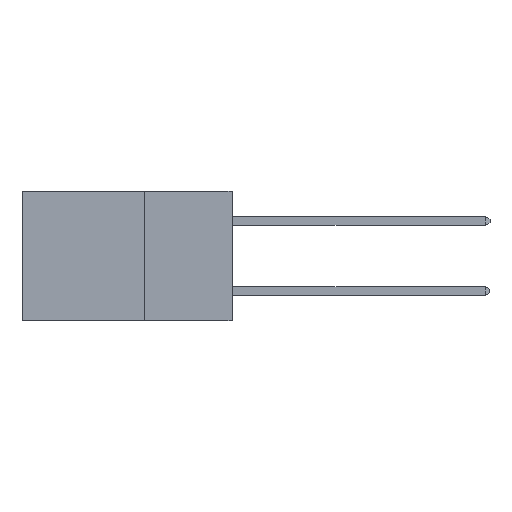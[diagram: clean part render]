
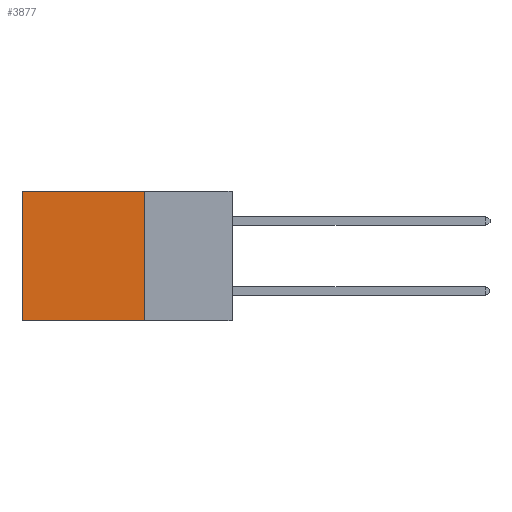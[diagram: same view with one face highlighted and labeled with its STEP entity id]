
A CAD part, left-side view. The second image highlights one B-rep face of the part: STEP entity #3877.
In plain terms, the highlighted planar face has unit normal (-1, 0, 0).
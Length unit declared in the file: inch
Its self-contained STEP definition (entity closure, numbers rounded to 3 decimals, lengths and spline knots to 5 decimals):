
#20 = VECTOR ( 'NONE', #9128, 39.37008 ) ;
#154 = VECTOR ( 'NONE', #14151, 39.37008 ) ;
#423 = LINE ( 'NONE', #7875, #20 ) ;
#1464 = ORIENTED_EDGE ( 'NONE', *, *, #12801, .F. ) ;
#1496 = EDGE_CURVE ( 'NONE', #2145, #12539, #3213, .T. ) ;
#2145 = VERTEX_POINT ( 'NONE', #14210 ) ;
#2491 = VECTOR ( 'NONE', #6498, 39.37008 ) ;
#3213 = LINE ( 'NONE', #7158, #15294 ) ;
#3415 = VERTEX_POINT ( 'NONE', #4336 ) ;
#3877 = ADVANCED_FACE ( 'NONE', ( #12768 ), #14203, .F. ) ;
#4336 = CARTESIAN_POINT ( 'NONE',  ( 0.2875, 0.25, 0. ) ) ;
#5233 = AXIS2_PLACEMENT_3D ( 'NONE', #11856, #15379, #8330 ) ;
#5775 = CARTESIAN_POINT ( 'NONE',  ( 0.2875, 0.6, 0. ) ) ;
#6446 = EDGE_CURVE ( 'NONE', #3415, #8809, #423, .T. ) ;
#6498 = DIRECTION ( 'NONE',  ( 0., 0., -1. ) ) ;
#7106 = DIRECTION ( 'NONE',  ( 0., 1., 0. ) ) ;
#7158 = CARTESIAN_POINT ( 'NONE',  ( 0.2875, 0.25, -0.37 ) ) ;
#7875 = CARTESIAN_POINT ( 'NONE',  ( 0.2875, 0.25, 0. ) ) ;
#8330 = DIRECTION ( 'NONE',  ( 0., 0., -1. ) ) ;
#8809 = VERTEX_POINT ( 'NONE', #14039 ) ;
#8878 = EDGE_CURVE ( 'NONE', #8809, #12539, #13314, .T. ) ;
#9128 = DIRECTION ( 'NONE',  ( 0., 1., 0. ) ) ;
#11319 = CARTESIAN_POINT ( 'NONE',  ( 0.2875, 0.25, 0. ) ) ;
#11384 = ORIENTED_EDGE ( 'NONE', *, *, #1496, .F. ) ;
#11856 = CARTESIAN_POINT ( 'NONE',  ( 0.2875, 0.25, 0. ) ) ;
#12539 = VERTEX_POINT ( 'NONE', #13288 ) ;
#12768 = FACE_OUTER_BOUND ( 'NONE', #15483, .T. ) ;
#12801 = EDGE_CURVE ( 'NONE', #3415, #2145, #15418, .T. ) ;
#13288 = CARTESIAN_POINT ( 'NONE',  ( 0.2875, 0.6, -0.37 ) ) ;
#13314 = LINE ( 'NONE', #5775, #154 ) ;
#14039 = CARTESIAN_POINT ( 'NONE',  ( 0.2875, 0.6, 0. ) ) ;
#14120 = ORIENTED_EDGE ( 'NONE', *, *, #6446, .T. ) ;
#14151 = DIRECTION ( 'NONE',  ( 0., 0., -1. ) ) ;
#14203 = PLANE ( 'NONE',  #5233 ) ;
#14210 = CARTESIAN_POINT ( 'NONE',  ( 0.2875, 0.25, -0.37 ) ) ;
#14860 = ORIENTED_EDGE ( 'NONE', *, *, #8878, .T. ) ;
#15294 = VECTOR ( 'NONE', #7106, 39.37008 ) ;
#15379 = DIRECTION ( 'NONE',  ( 1., 0., 0. ) ) ;
#15418 = LINE ( 'NONE', #11319, #2491 ) ;
#15483 = EDGE_LOOP ( 'NONE', ( #14860, #11384, #1464, #14120 ) ) ;
